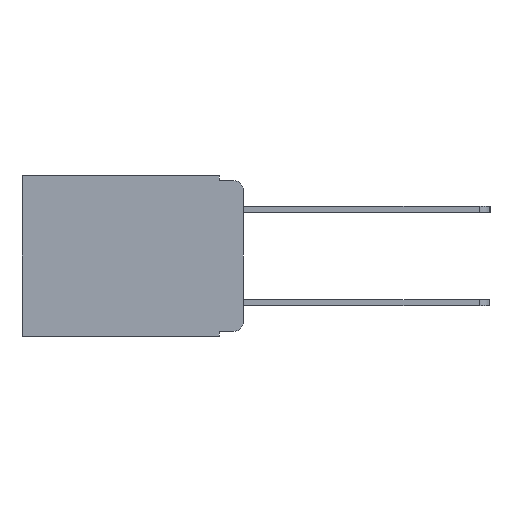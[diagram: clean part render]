
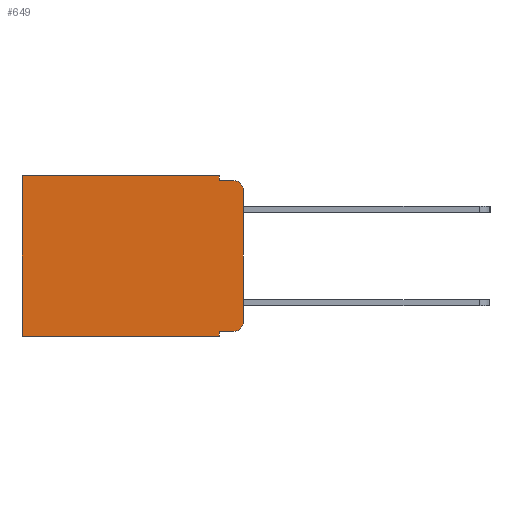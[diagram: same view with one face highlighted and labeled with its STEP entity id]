
A CAD part, left-side view. The second image highlights one B-rep face of the part: STEP entity #649.
In plain terms, the highlighted planar face has unit normal (-1, 0, 0).
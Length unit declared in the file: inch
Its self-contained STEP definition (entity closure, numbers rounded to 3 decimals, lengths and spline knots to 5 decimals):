
#6 = ORIENTED_EDGE ( 'NONE', *, *, #12107, .T. ) ;
#649 = ADVANCED_FACE ( 'NONE', ( #20580 ), #2067, .F. ) ;
#701 = CARTESIAN_POINT ( 'NONE',  ( 0.298, 0.02, -0.333 ) ) ;
#787 = DIRECTION ( 'NONE',  ( 0., -1., 0. ) ) ;
#1300 = ORIENTED_EDGE ( 'NONE', *, *, #9645, .F. ) ;
#1604 = CARTESIAN_POINT ( 'NONE',  ( 0.298, 0.051, 0. ) ) ;
#2048 = DIRECTION ( 'NONE',  ( 0., 0., -1. ) ) ;
#2067 = PLANE ( 'NONE',  #5120 ) ;
#2119 = LINE ( 'NONE', #3304, #10966 ) ;
#2190 = DIRECTION ( 'NONE',  ( 0., 0., -1. ) ) ;
#2413 = CARTESIAN_POINT ( 'NONE',  ( 0.298, 0.051, -0.01 ) ) ;
#3211 = CARTESIAN_POINT ( 'NONE',  ( 0.298, 0.02, -0.313 ) ) ;
#3246 = VERTEX_POINT ( 'NONE', #9570 ) ;
#3304 = CARTESIAN_POINT ( 'NONE',  ( 0.298, 0., -0.343 ) ) ;
#3386 = VERTEX_POINT ( 'NONE', #5233 ) ;
#3611 = CARTESIAN_POINT ( 'NONE',  ( 0.298, 0., 0. ) ) ;
#3668 = LINE ( 'NONE', #4405, #8654 ) ;
#3738 = DIRECTION ( 'NONE',  ( 0., -1., 0. ) ) ;
#4235 = CARTESIAN_POINT ( 'NONE',  ( 0.298, 0.051, -0.333 ) ) ;
#4238 = VECTOR ( 'NONE', #3738, 39.37008 ) ;
#4405 = CARTESIAN_POINT ( 'NONE',  ( 0.298, 0.473, 0. ) ) ;
#4893 = DIRECTION ( 'NONE',  ( 0., 0., -1. ) ) ;
#5120 = AXIS2_PLACEMENT_3D ( 'NONE', #10113, #11907, #2190 ) ;
#5128 = VECTOR ( 'NONE', #16398, 39.37008 ) ;
#5233 = CARTESIAN_POINT ( 'NONE',  ( 0.298, 0.02, -0.01 ) ) ;
#5297 = VERTEX_POINT ( 'NONE', #701 ) ;
#5314 = LINE ( 'NONE', #8802, #4238 ) ;
#5342 = EDGE_CURVE ( 'NONE', #18188, #8561, #19451, .T. ) ;
#6053 = DIRECTION ( 'NONE',  ( 0., 0., -1. ) ) ;
#6256 = VECTOR ( 'NONE', #2048, 39.37008 ) ;
#6389 = EDGE_CURVE ( 'NONE', #17221, #5297, #5314, .T. ) ;
#6912 = ORIENTED_EDGE ( 'NONE', *, *, #6389, .T. ) ;
#7078 = CARTESIAN_POINT ( 'NONE',  ( 0.298, 0., -0.03 ) ) ;
#7382 = EDGE_CURVE ( 'NONE', #11189, #20000, #2119, .T. ) ;
#7983 = EDGE_CURVE ( 'NONE', #5297, #8561, #16516, .T. ) ;
#8406 = ORIENTED_EDGE ( 'NONE', *, *, #12495, .T. ) ;
#8561 = VERTEX_POINT ( 'NONE', #11313 ) ;
#8627 = CARTESIAN_POINT ( 'NONE',  ( 0.298, 0.473, -0.343 ) ) ;
#8654 = VECTOR ( 'NONE', #6053, 39.37008 ) ;
#8802 = CARTESIAN_POINT ( 'NONE',  ( 0.298, 0.051, -0.333 ) ) ;
#9570 = CARTESIAN_POINT ( 'NONE',  ( 0.298, 0.473, 0. ) ) ;
#9645 = EDGE_CURVE ( 'NONE', #15911, #3386, #15445, .T. ) ;
#9668 = DIRECTION ( 'NONE',  ( -1., 0., 0. ) ) ;
#10113 = CARTESIAN_POINT ( 'NONE',  ( 0.298, 0., 0. ) ) ;
#10287 = EDGE_LOOP ( 'NONE', ( #13509, #8406, #1300, #16287, #6, #18945, #20198, #13306, #6912, #18918 ) ) ;
#10661 = LINE ( 'NONE', #16815, #6256 ) ;
#10865 = EDGE_CURVE ( 'NONE', #15614, #15911, #13846, .T. ) ;
#10966 = VECTOR ( 'NONE', #14811, 39.37008 ) ;
#11139 = VECTOR ( 'NONE', #787, 39.37008 ) ;
#11189 = VERTEX_POINT ( 'NONE', #15653 ) ;
#11313 = CARTESIAN_POINT ( 'NONE',  ( 0.298, 0., -0.313 ) ) ;
#11821 = LINE ( 'NONE', #3611, #12328 ) ;
#11907 = DIRECTION ( 'NONE',  ( 1., 0., 0. ) ) ;
#12107 = EDGE_CURVE ( 'NONE', #15614, #3246, #11821, .T. ) ;
#12328 = VECTOR ( 'NONE', #15123, 39.37008 ) ;
#12329 = CARTESIAN_POINT ( 'NONE',  ( 0.298, 0.051, -0.01 ) ) ;
#12495 = EDGE_CURVE ( 'NONE', #18188, #3386, #12806, .T. ) ;
#12806 = CIRCLE ( 'NONE', #15376, 0.02 ) ;
#12866 = CARTESIAN_POINT ( 'NONE',  ( 0.298, 0.051, 0. ) ) ;
#13306 = ORIENTED_EDGE ( 'NONE', *, *, #15710, .F. ) ;
#13328 = AXIS2_PLACEMENT_3D ( 'NONE', #3211, #14716, #4893 ) ;
#13509 = ORIENTED_EDGE ( 'NONE', *, *, #5342, .F. ) ;
#13846 = LINE ( 'NONE', #1604, #5128 ) ;
#14716 = DIRECTION ( 'NONE',  ( -1., 0., 0. ) ) ;
#14811 = DIRECTION ( 'NONE',  ( 0., 1., 0. ) ) ;
#15085 = VECTOR ( 'NONE', #17606, 39.37008 ) ;
#15123 = DIRECTION ( 'NONE',  ( 0., 1., 0. ) ) ;
#15376 = AXIS2_PLACEMENT_3D ( 'NONE', #19409, #9668, #21015 ) ;
#15445 = LINE ( 'NONE', #2413, #11139 ) ;
#15614 = VERTEX_POINT ( 'NONE', #12866 ) ;
#15653 = CARTESIAN_POINT ( 'NONE',  ( 0.298, 0.051, -0.343 ) ) ;
#15710 = EDGE_CURVE ( 'NONE', #17221, #11189, #10661, .T. ) ;
#15911 = VERTEX_POINT ( 'NONE', #12329 ) ;
#16287 = ORIENTED_EDGE ( 'NONE', *, *, #10865, .F. ) ;
#16398 = DIRECTION ( 'NONE',  ( 0., 0., -1. ) ) ;
#16516 = CIRCLE ( 'NONE', #13328, 0.02 ) ;
#16815 = CARTESIAN_POINT ( 'NONE',  ( 0.298, 0.051, 0. ) ) ;
#17221 = VERTEX_POINT ( 'NONE', #4235 ) ;
#17606 = DIRECTION ( 'NONE',  ( 0., 0., -1. ) ) ;
#18188 = VERTEX_POINT ( 'NONE', #7078 ) ;
#18918 = ORIENTED_EDGE ( 'NONE', *, *, #7983, .T. ) ;
#18945 = ORIENTED_EDGE ( 'NONE', *, *, #19016, .T. ) ;
#19016 = EDGE_CURVE ( 'NONE', #3246, #20000, #3668, .T. ) ;
#19409 = CARTESIAN_POINT ( 'NONE',  ( 0.298, 0.02, -0.03 ) ) ;
#19451 = LINE ( 'NONE', #20496, #15085 ) ;
#20000 = VERTEX_POINT ( 'NONE', #8627 ) ;
#20198 = ORIENTED_EDGE ( 'NONE', *, *, #7382, .F. ) ;
#20496 = CARTESIAN_POINT ( 'NONE',  ( 0.298, 0., 0. ) ) ;
#20580 = FACE_OUTER_BOUND ( 'NONE', #10287, .T. ) ;
#21015 = DIRECTION ( 'NONE',  ( 0., 0., -1. ) ) ;
